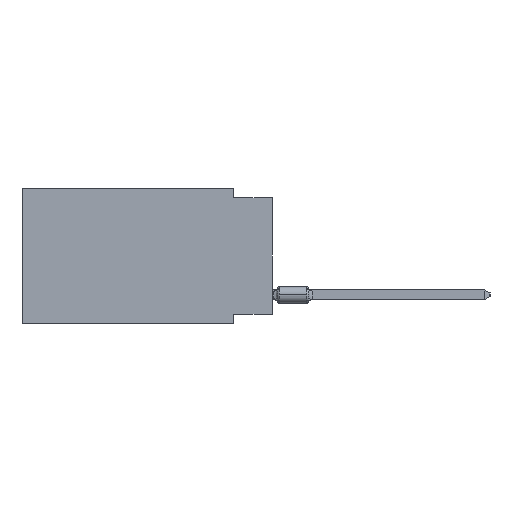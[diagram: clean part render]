
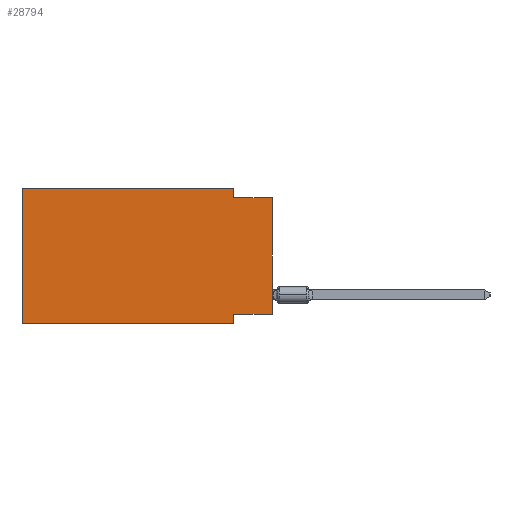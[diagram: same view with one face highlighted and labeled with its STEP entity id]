
A CAD part, left-side view. The second image highlights one B-rep face of the part: STEP entity #28794.
In plain terms, the highlighted planar face has unit normal (-1, 0, 0).
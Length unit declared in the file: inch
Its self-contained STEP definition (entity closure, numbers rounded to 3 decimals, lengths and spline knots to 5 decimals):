
#483 = DIRECTION ( 'NONE',  ( 0., -1., 0. ) ) ;
#1663 = CARTESIAN_POINT ( 'NONE',  ( 0., 0.1, 0. ) ) ;
#1937 = VECTOR ( 'NONE', #8820, 39.37008 ) ;
#2468 = ORIENTED_EDGE ( 'NONE', *, *, #16479, .F. ) ;
#2902 = EDGE_LOOP ( 'NONE', ( #14192, #2468, #44712, #32957, #5059, #58930, #60324, #40078 ) ) ;
#3326 = LINE ( 'NONE', #34782, #5442 ) ;
#3533 = DIRECTION ( 'NONE',  ( 0., -1., 0. ) ) ;
#5059 = ORIENTED_EDGE ( 'NONE', *, *, #31510, .F. ) ;
#5156 = DIRECTION ( 'NONE',  ( 1., 0., 0. ) ) ;
#5442 = VECTOR ( 'NONE', #29307, 39.37008 ) ;
#5815 = EDGE_CURVE ( 'NONE', #36316, #52162, #47343, .T. ) ;
#8820 = DIRECTION ( 'NONE',  ( 0., 1., 0. ) ) ;
#8959 = LINE ( 'NONE', #45899, #62184 ) ;
#10621 = CARTESIAN_POINT ( 'NONE',  ( 0., 0.645, 0. ) ) ;
#11152 = EDGE_CURVE ( 'NONE', #65148, #13010, #22119, .T. ) ;
#13010 = VERTEX_POINT ( 'NONE', #40253 ) ;
#13611 = CARTESIAN_POINT ( 'NONE',  ( 0., 0., -0.325 ) ) ;
#14192 = ORIENTED_EDGE ( 'NONE', *, *, #18987, .T. ) ;
#15943 = DIRECTION ( 'NONE',  ( 0., 0., -1. ) ) ;
#16479 = EDGE_CURVE ( 'NONE', #26781, #55175, #19245, .T. ) ;
#16804 = EDGE_CURVE ( 'NONE', #66223, #65148, #30351, .T. ) ;
#16934 = CARTESIAN_POINT ( 'NONE',  ( 0., 0.645, -0.35 ) ) ;
#18987 = EDGE_CURVE ( 'NONE', #66223, #55175, #3326, .T. ) ;
#19245 = LINE ( 'NONE', #39771, #56514 ) ;
#20465 = CARTESIAN_POINT ( 'NONE',  ( 0., 0., -0.325 ) ) ;
#21110 = EDGE_CURVE ( 'NONE', #65158, #13010, #49105, .T. ) ;
#22119 = LINE ( 'NONE', #47777, #56191 ) ;
#23082 = CARTESIAN_POINT ( 'NONE',  ( 0., 0.1, -0.325 ) ) ;
#23088 = CARTESIAN_POINT ( 'NONE',  ( 0., 0.645, -0.35 ) ) ;
#26781 = VERTEX_POINT ( 'NONE', #40037 ) ;
#27378 = DIRECTION ( 'NONE',  ( 0., 0., -1. ) ) ;
#27647 = CARTESIAN_POINT ( 'NONE',  ( 0., 0., -0.025 ) ) ;
#28794 = ADVANCED_FACE ( 'NONE', ( #57484 ), #63303, .F. ) ;
#29307 = DIRECTION ( 'NONE',  ( 0., 0., 1. ) ) ;
#30351 = LINE ( 'NONE', #13611, #1937 ) ;
#31510 = EDGE_CURVE ( 'NONE', #65158, #36316, #8959, .T. ) ;
#32532 = DIRECTION ( 'NONE',  ( 0., 0., -1. ) ) ;
#32957 = ORIENTED_EDGE ( 'NONE', *, *, #5815, .F. ) ;
#34782 = CARTESIAN_POINT ( 'NONE',  ( 0., 0., 0. ) ) ;
#36316 = VERTEX_POINT ( 'NONE', #40725 ) ;
#37595 = VECTOR ( 'NONE', #483, 39.37008 ) ;
#39771 = CARTESIAN_POINT ( 'NONE',  ( 0., 0., -0.025 ) ) ;
#40037 = CARTESIAN_POINT ( 'NONE',  ( 0., 0.1, -0.025 ) ) ;
#40078 = ORIENTED_EDGE ( 'NONE', *, *, #16804, .F. ) ;
#40253 = CARTESIAN_POINT ( 'NONE',  ( 0., 0.1, -0.35 ) ) ;
#40725 = CARTESIAN_POINT ( 'NONE',  ( 0., 0.645, 0. ) ) ;
#43756 = VECTOR ( 'NONE', #32532, 39.37008 ) ;
#43937 = DIRECTION ( 'NONE',  ( 0., -1., 0. ) ) ;
#44712 = ORIENTED_EDGE ( 'NONE', *, *, #51081, .F. ) ;
#45577 = AXIS2_PLACEMENT_3D ( 'NONE', #10621, #5156, #27378 ) ;
#45899 = CARTESIAN_POINT ( 'NONE',  ( 0., 0.645, 0. ) ) ;
#46467 = VECTOR ( 'NONE', #43937, 39.37008 ) ;
#47343 = LINE ( 'NONE', #58277, #37595 ) ;
#47777 = CARTESIAN_POINT ( 'NONE',  ( 0., 0.1, -0.35 ) ) ;
#49105 = LINE ( 'NONE', #23088, #46467 ) ;
#51081 = EDGE_CURVE ( 'NONE', #52162, #26781, #57514, .T. ) ;
#52076 = CARTESIAN_POINT ( 'NONE',  ( 0., 0.1, 0. ) ) ;
#52162 = VERTEX_POINT ( 'NONE', #1663 ) ;
#55175 = VERTEX_POINT ( 'NONE', #27647 ) ;
#55825 = DIRECTION ( 'NONE',  ( 0., 0., 1. ) ) ;
#56191 = VECTOR ( 'NONE', #15943, 39.37008 ) ;
#56514 = VECTOR ( 'NONE', #3533, 39.37008 ) ;
#57484 = FACE_OUTER_BOUND ( 'NONE', #2902, .T. ) ;
#57514 = LINE ( 'NONE', #52076, #43756 ) ;
#58277 = CARTESIAN_POINT ( 'NONE',  ( 0., 0.645, 0. ) ) ;
#58930 = ORIENTED_EDGE ( 'NONE', *, *, #21110, .T. ) ;
#60324 = ORIENTED_EDGE ( 'NONE', *, *, #11152, .F. ) ;
#62184 = VECTOR ( 'NONE', #55825, 39.37008 ) ;
#63303 = PLANE ( 'NONE',  #45577 ) ;
#65148 = VERTEX_POINT ( 'NONE', #23082 ) ;
#65158 = VERTEX_POINT ( 'NONE', #16934 ) ;
#66223 = VERTEX_POINT ( 'NONE', #20465 ) ;
